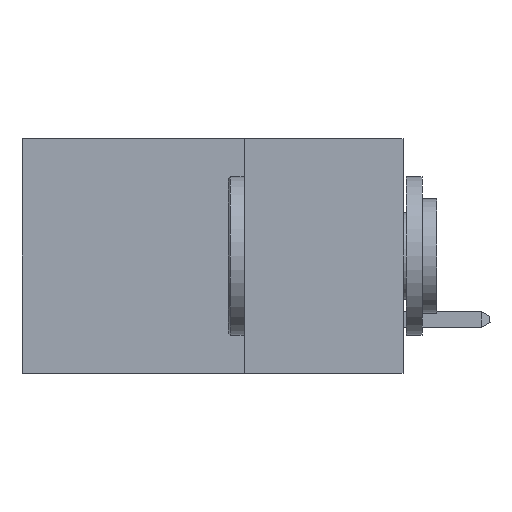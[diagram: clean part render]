
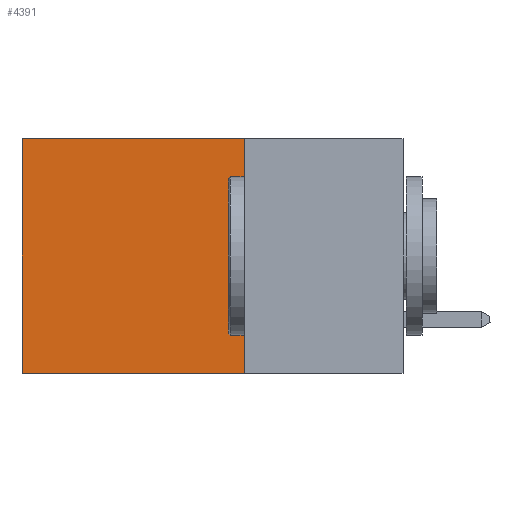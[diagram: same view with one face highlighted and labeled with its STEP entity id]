
A CAD part, left-side view. The second image highlights one B-rep face of the part: STEP entity #4391.
In plain terms, the highlighted planar face has unit normal (-1, 0, 0).
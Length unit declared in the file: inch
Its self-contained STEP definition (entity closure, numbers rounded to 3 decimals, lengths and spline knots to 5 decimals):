
#489 = PLANE ( 'NONE',  #4687 ) ;
#1091 = VECTOR ( 'NONE', #3988, 39.37008 ) ;
#1113 = VECTOR ( 'NONE', #6193, 39.37008 ) ;
#2182 = CARTESIAN_POINT ( 'NONE',  ( 0.2875, 0.25, 0. ) ) ;
#2263 = DIRECTION ( 'NONE',  ( 1., 0., 0. ) ) ;
#3625 = LINE ( 'NONE', #13846, #12832 ) ;
#3988 = DIRECTION ( 'NONE',  ( 0., 0., -1. ) ) ;
#4335 = CARTESIAN_POINT ( 'NONE',  ( 0.2875, 0.25, 0. ) ) ;
#4391 = ADVANCED_FACE ( 'NONE', ( #14661 ), #489, .F. ) ;
#4687 = AXIS2_PLACEMENT_3D ( 'NONE', #2182, #2263, #14360 ) ;
#5070 = EDGE_CURVE ( 'NONE', #7681, #6936, #10300, .T. ) ;
#5754 = ORIENTED_EDGE ( 'NONE', *, *, #14419, .F. ) ;
#6193 = DIRECTION ( 'NONE',  ( 0., 1., 0. ) ) ;
#6353 = CARTESIAN_POINT ( 'NONE',  ( 0.2875, 0.25, 0. ) ) ;
#6936 = VERTEX_POINT ( 'NONE', #14189 ) ;
#7151 = EDGE_CURVE ( 'NONE', #12409, #6936, #19485, .T. ) ;
#7681 = VERTEX_POINT ( 'NONE', #14543 ) ;
#8682 = EDGE_LOOP ( 'NONE', ( #17777, #17399, #5754, #11375 ) ) ;
#10300 = LINE ( 'NONE', #17805, #1091 ) ;
#11049 = VECTOR ( 'NONE', #18421, 39.37008 ) ;
#11322 = CARTESIAN_POINT ( 'NONE',  ( 0.2875, 0.25, -0.37 ) ) ;
#11375 = ORIENTED_EDGE ( 'NONE', *, *, #11896, .T. ) ;
#11896 = EDGE_CURVE ( 'NONE', #19121, #7681, #3625, .T. ) ;
#12409 = VERTEX_POINT ( 'NONE', #20287 ) ;
#12832 = VECTOR ( 'NONE', #15578, 39.37008 ) ;
#13846 = CARTESIAN_POINT ( 'NONE',  ( 0.2875, 0.25, 0. ) ) ;
#14189 = CARTESIAN_POINT ( 'NONE',  ( 0.2875, 0.6, -0.37 ) ) ;
#14360 = DIRECTION ( 'NONE',  ( 0., 0., -1. ) ) ;
#14419 = EDGE_CURVE ( 'NONE', #19121, #12409, #15121, .T. ) ;
#14543 = CARTESIAN_POINT ( 'NONE',  ( 0.2875, 0.6, 0. ) ) ;
#14661 = FACE_OUTER_BOUND ( 'NONE', #8682, .T. ) ;
#15121 = LINE ( 'NONE', #6353, #11049 ) ;
#15578 = DIRECTION ( 'NONE',  ( 0., 1., 0. ) ) ;
#17399 = ORIENTED_EDGE ( 'NONE', *, *, #7151, .F. ) ;
#17777 = ORIENTED_EDGE ( 'NONE', *, *, #5070, .T. ) ;
#17805 = CARTESIAN_POINT ( 'NONE',  ( 0.2875, 0.6, 0. ) ) ;
#18421 = DIRECTION ( 'NONE',  ( 0., 0., -1. ) ) ;
#19121 = VERTEX_POINT ( 'NONE', #4335 ) ;
#19485 = LINE ( 'NONE', #11322, #1113 ) ;
#20287 = CARTESIAN_POINT ( 'NONE',  ( 0.2875, 0.25, -0.37 ) ) ;
